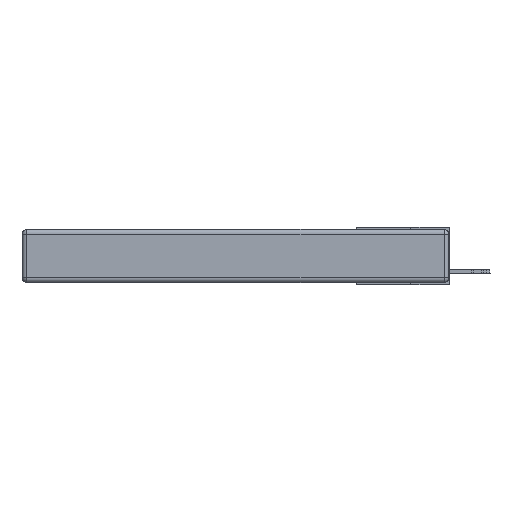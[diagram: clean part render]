
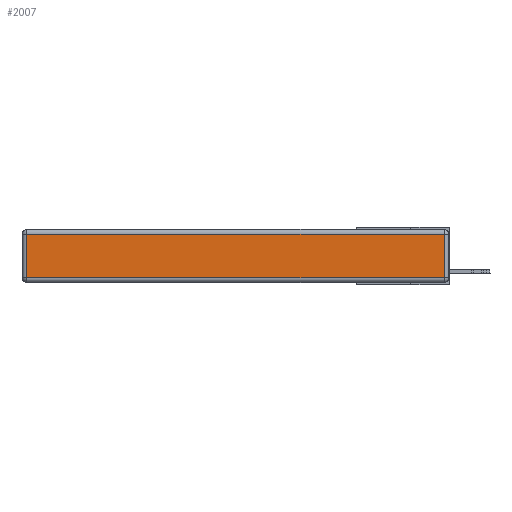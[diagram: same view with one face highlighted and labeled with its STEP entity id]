
A CAD part, left-side view. The second image highlights one B-rep face of the part: STEP entity #2007.
In plain terms, the highlighted planar face has unit normal (-1, 0, 0).
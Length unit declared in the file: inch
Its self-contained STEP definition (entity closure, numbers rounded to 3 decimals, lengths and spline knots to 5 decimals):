
#902 = LINE ( 'NONE', #2369, #3486 ) ;
#1684 = CARTESIAN_POINT ( 'NONE',  ( 0., 0.03, -0.313 ) ) ;
#1695 = VERTEX_POINT ( 'NONE', #1684 ) ;
#2007 = ADVANCED_FACE ( 'NONE', ( #3961 ), #22140, .T. ) ;
#2369 = CARTESIAN_POINT ( 'NONE',  ( 0., 2.72, -0.343 ) ) ;
#2540 = ORIENTED_EDGE ( 'NONE', *, *, #12810, .T. ) ;
#3486 = VECTOR ( 'NONE', #15738, 39.37008 ) ;
#3961 = FACE_OUTER_BOUND ( 'NONE', #11421, .T. ) ;
#4981 = VECTOR ( 'NONE', #28442, 39.37008 ) ;
#5419 = CARTESIAN_POINT ( 'NONE',  ( 0., 0., -0.313 ) ) ;
#5710 = LINE ( 'NONE', #5419, #4981 ) ;
#6479 = CARTESIAN_POINT ( 'NONE',  ( 0., 0.03, -0.03 ) ) ;
#7563 = LINE ( 'NONE', #21570, #17438 ) ;
#8714 = VERTEX_POINT ( 'NONE', #23334 ) ;
#9013 = CARTESIAN_POINT ( 'NONE',  ( 0., 2.72, -0.313 ) ) ;
#11421 = EDGE_LOOP ( 'NONE', ( #28354, #26954, #14749, #2540 ) ) ;
#11713 = CARTESIAN_POINT ( 'NONE',  ( 0., 0.03, -0.343 ) ) ;
#12454 = DIRECTION ( 'NONE',  ( -1., 0., 0. ) ) ;
#12810 = EDGE_CURVE ( 'NONE', #8714, #29479, #902, .T. ) ;
#14038 = DIRECTION ( 'NONE',  ( 0., 0., 1. ) ) ;
#14749 = ORIENTED_EDGE ( 'NONE', *, *, #16960, .T. ) ;
#15738 = DIRECTION ( 'NONE',  ( 0., 0., -1. ) ) ;
#16790 = DIRECTION ( 'NONE',  ( 0., 1., 0. ) ) ;
#16960 = EDGE_CURVE ( 'NONE', #29507, #8714, #7563, .T. ) ;
#17090 = AXIS2_PLACEMENT_3D ( 'NONE', #17448, #12454, #26428 ) ;
#17438 = VECTOR ( 'NONE', #16790, 39.37008 ) ;
#17448 = CARTESIAN_POINT ( 'NONE',  ( 0., 0., -0.343 ) ) ;
#18006 = LINE ( 'NONE', #11713, #23504 ) ;
#18145 = EDGE_CURVE ( 'NONE', #29479, #1695, #5710, .T. ) ;
#21570 = CARTESIAN_POINT ( 'NONE',  ( 0., 2.75, -0.03 ) ) ;
#22140 = PLANE ( 'NONE',  #17090 ) ;
#23334 = CARTESIAN_POINT ( 'NONE',  ( 0., 2.72, -0.03 ) ) ;
#23504 = VECTOR ( 'NONE', #14038, 39.37008 ) ;
#26428 = DIRECTION ( 'NONE',  ( 0., 0., 1. ) ) ;
#26954 = ORIENTED_EDGE ( 'NONE', *, *, #30209, .T. ) ;
#28354 = ORIENTED_EDGE ( 'NONE', *, *, #18145, .T. ) ;
#28442 = DIRECTION ( 'NONE',  ( 0., -1., 0. ) ) ;
#29479 = VERTEX_POINT ( 'NONE', #9013 ) ;
#29507 = VERTEX_POINT ( 'NONE', #6479 ) ;
#30209 = EDGE_CURVE ( 'NONE', #1695, #29507, #18006, .T. ) ;
